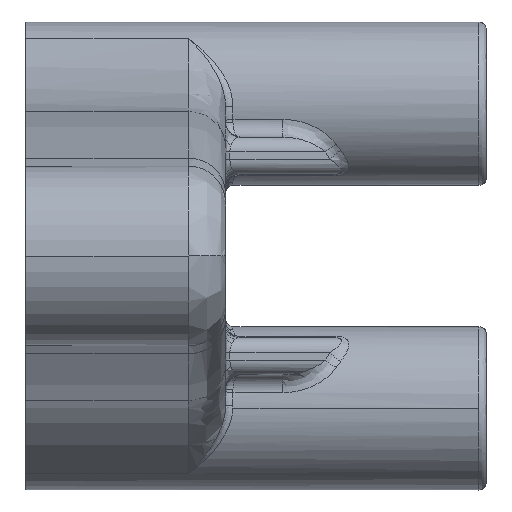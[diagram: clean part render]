
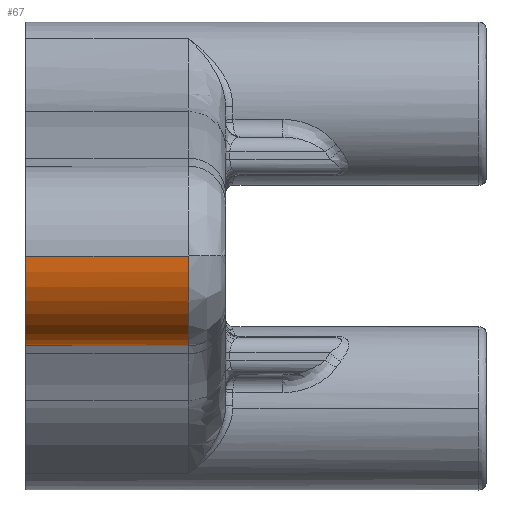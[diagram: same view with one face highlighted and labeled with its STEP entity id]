
A CAD part, front view. The second image highlights one B-rep face of the part: STEP entity #67.
In plain terms, the highlighted cylindrical face has radius 12.15 mm (diameter 24.3 mm), a partial arc.
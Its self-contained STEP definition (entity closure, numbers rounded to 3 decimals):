
#67 = ADVANCED_FACE ( 'NONE', ( #3851 ), #4812, .T. ) ;
#227 = DIRECTION ( 'NONE',  ( -1., 0., 0. ) ) ;
#353 = ORIENTED_EDGE ( 'NONE', *, *, #5617, .T. ) ;
#1023 = AXIS2_PLACEMENT_3D ( 'NONE', #1073, #4699, #2769 ) ;
#1073 = CARTESIAN_POINT ( 'NONE',  ( -431.682, -86.722, 1.048 ) ) ;
#1530 = CARTESIAN_POINT ( 'NONE',  ( -409.782, -98.872, 1. ) ) ;
#1934 = EDGE_CURVE ( 'NONE', #4551, #4485, #4050, .T. ) ;
#2010 = CARTESIAN_POINT ( 'NONE',  ( -431.682, -98.872, 1. ) ) ;
#2084 = VERTEX_POINT ( 'NONE', #4566 ) ;
#2161 = AXIS2_PLACEMENT_3D ( 'NONE', #2872, #5269, #2353 ) ;
#2353 = DIRECTION ( 'NONE',  ( 0., -1., 0. ) ) ;
#2608 = DIRECTION ( 'NONE',  ( -1., 0., 0. ) ) ;
#2681 = DIRECTION ( 'NONE',  ( 0., -1., 0. ) ) ;
#2695 = EDGE_CURVE ( 'NONE', #6380, #3337, #3534, .T. ) ;
#2769 = DIRECTION ( 'NONE',  ( 0., -1., 0. ) ) ;
#2778 = CARTESIAN_POINT ( 'NONE',  ( -431.682, -84.74, -10.939 ) ) ;
#2872 = CARTESIAN_POINT ( 'NONE',  ( -404.682, -86.722, 1.048 ) ) ;
#2933 = ORIENTED_EDGE ( 'NONE', *, *, #1934, .T. ) ;
#3337 = VERTEX_POINT ( 'NONE', #1530 ) ;
#3534 = CIRCLE ( 'NONE', #4290, 12.15 ) ;
#3577 = DIRECTION ( 'NONE',  ( 0., -1., 0. ) ) ;
#3663 = CARTESIAN_POINT ( 'NONE',  ( -404.682, -84.74, -10.939 ) ) ;
#3813 = EDGE_CURVE ( 'NONE', #3337, #4551, #4695, .T. ) ;
#3840 = CARTESIAN_POINT ( 'NONE',  ( -404.682, -98.872, 1. ) ) ;
#3851 = FACE_OUTER_BOUND ( 'NONE', #4333, .T. ) ;
#3902 = ORIENTED_EDGE ( 'NONE', *, *, #4275, .T. ) ;
#3977 = VECTOR ( 'NONE', #227, 1000. ) ;
#4050 = CIRCLE ( 'NONE', #1023, 12.15 ) ;
#4059 = CARTESIAN_POINT ( 'NONE',  ( -409.782, -86.722, -11.102 ) ) ;
#4085 = ORIENTED_EDGE ( 'NONE', *, *, #2695, .T. ) ;
#4090 = AXIS2_PLACEMENT_3D ( 'NONE', #4228, #5699, #2681 ) ;
#4200 = LINE ( 'NONE', #3663, #5971 ) ;
#4228 = CARTESIAN_POINT ( 'NONE',  ( -409.782, -86.722, 1.048 ) ) ;
#4275 = EDGE_CURVE ( 'NONE', #4485, #2084, #4200, .T. ) ;
#4290 = AXIS2_PLACEMENT_3D ( 'NONE', #5164, #2608, #3577 ) ;
#4333 = EDGE_LOOP ( 'NONE', ( #2933, #3902, #353, #4085, #5081 ) ) ;
#4485 = VERTEX_POINT ( 'NONE', #2778 ) ;
#4551 = VERTEX_POINT ( 'NONE', #2010 ) ;
#4566 = CARTESIAN_POINT ( 'NONE',  ( -409.782, -84.74, -10.939 ) ) ;
#4695 = LINE ( 'NONE', #3840, #3977 ) ;
#4699 = DIRECTION ( 'NONE',  ( 1., 0., 0. ) ) ;
#4812 = CYLINDRICAL_SURFACE ( 'NONE', #2161, 12.15 ) ;
#5081 = ORIENTED_EDGE ( 'NONE', *, *, #3813, .T. ) ;
#5164 = CARTESIAN_POINT ( 'NONE',  ( -409.782, -86.722, 1.048 ) ) ;
#5269 = DIRECTION ( 'NONE',  ( -1., 0., 0. ) ) ;
#5282 = DIRECTION ( 'NONE',  ( 1., 0., 0. ) ) ;
#5617 = EDGE_CURVE ( 'NONE', #2084, #6380, #6079, .T. ) ;
#5699 = DIRECTION ( 'NONE',  ( -1., 0., 0. ) ) ;
#5971 = VECTOR ( 'NONE', #5282, 1000. ) ;
#6079 = CIRCLE ( 'NONE', #4090, 12.15 ) ;
#6380 = VERTEX_POINT ( 'NONE', #4059 ) ;
